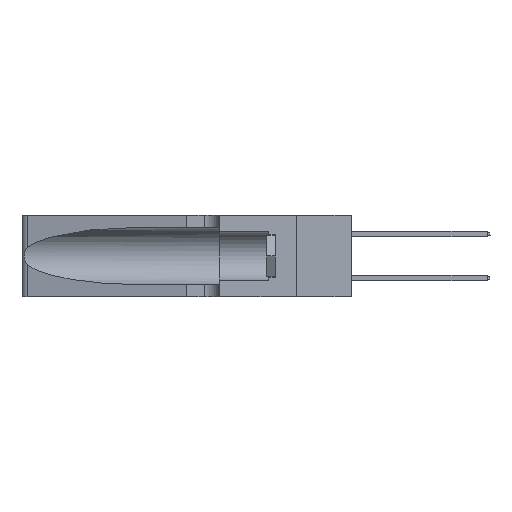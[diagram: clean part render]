
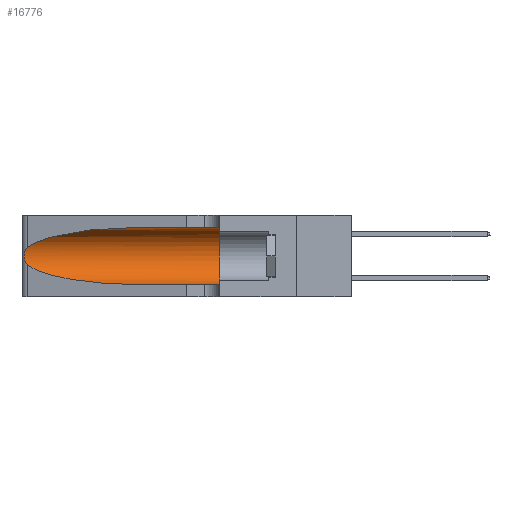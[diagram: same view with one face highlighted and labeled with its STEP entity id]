
A CAD part, left-side view. The second image highlights one B-rep face of the part: STEP entity #16776.
In plain terms, the highlighted cylindrical face has radius 3.308 mm (diameter 6.617 mm), a partial arc.
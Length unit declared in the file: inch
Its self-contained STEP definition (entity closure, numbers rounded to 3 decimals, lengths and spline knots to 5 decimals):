
#282 = EDGE_LOOP ( 'NONE', ( #28429, #18808, #9263, #42537, #4677, #20917 ) ) ;
#328 = CARTESIAN_POINT ( 'NONE',  ( 0.2373, 1.15595, 0.28018 ) ) ;
#1900 = CARTESIAN_POINT ( 'NONE',  ( 0.25487, 1.22718, 0.22369 ) ) ;
#2048 = CARTESIAN_POINT ( 'NONE',  ( 0.25787, 1.23484, 0.2124 ) ) ;
#2056 = VERTEX_POINT ( 'NONE', #17497 ) ;
#2683 = VECTOR ( 'NONE', #10957, 39.37008 ) ;
#3288 = CARTESIAN_POINT ( 'NONE',  ( 0.1305, 1.61858, 0.31525 ) ) ;
#4677 = ORIENTED_EDGE ( 'NONE', *, *, #41355, .F. ) ;
#5514 = CARTESIAN_POINT ( 'NONE',  ( 0.26018, 1.23835, 0.19895 ) ) ;
#6188 = CARTESIAN_POINT ( 'NONE',  ( 0.1305, 0.72297, 0.31525 ) ) ;
#6621 = DIRECTION ( 'NONE',  ( 0., 0., -1. ) ) ;
#8950 = CARTESIAN_POINT ( 'NONE',  ( 0.26075, 1.23896, 0.178 ) ) ;
#9249 = CARTESIAN_POINT ( 'NONE',  ( 0.25487, 1.22718, 0.14631 ) ) ;
#9263 = ORIENTED_EDGE ( 'NONE', *, *, #12343, .T. ) ;
#10132 = CARTESIAN_POINT ( 'NONE',  ( 0.25487, 1.22718, 0.14631 ) ) ;
#10921 = DIRECTION ( 'NONE',  ( 0., 1., 0. ) ) ;
#10957 = DIRECTION ( 'NONE',  ( 0., -1., 0. ) ) ;
#11617 = CARTESIAN_POINT ( 'NONE',  ( 0.1305, 0.35, 0.05475 ) ) ;
#12343 = EDGE_CURVE ( 'NONE', #20862, #30946, #29316, .T. ) ;
#12430 = CARTESIAN_POINT ( 'NONE',  ( 0.25856, 1.23593, 0.16098 ) ) ;
#13592 = CARTESIAN_POINT ( 'NONE',  ( 0.18966, 0.96281, 0.05475 ) ) ;
#14244 = CARTESIAN_POINT ( 'NONE',  ( 0.1305, 0.72297, 0.05475 ) ) ;
#15892 = CARTESIAN_POINT ( 'NONE',  ( 0.25639, 1.23186, 0.15144 ) ) ;
#16776 = ADVANCED_FACE ( 'NONE', ( #23261 ), #31228, .F. ) ;
#17061 = CARTESIAN_POINT ( 'NONE',  ( 0.1305, 0.72297, 0.05475 ) ) ;
#17246 = VECTOR ( 'NONE', #27312, 39.37008 ) ;
#17471 = CARTESIAN_POINT ( 'NONE',  ( 0.18966, 0.96281, 0.31525 ) ) ;
#17497 = CARTESIAN_POINT ( 'NONE',  ( 0.1305, 0.35, 0.31525 ) ) ;
#18808 = ORIENTED_EDGE ( 'NONE', *, *, #31252, .T. ) ;
#19390 = CARTESIAN_POINT ( 'NONE',  ( 0.25487, 1.22718, 0.14631 ) ) ;
#19931 = LINE ( 'NONE', #31491, #2683 ) ;
#20267 = EDGE_CURVE ( 'NONE', #30145, #40987, #33927, .T. ) ;
#20862 = VERTEX_POINT ( 'NONE', #9249 ) ;
#20917 = ORIENTED_EDGE ( 'NONE', *, *, #39255, .F. ) ;
#22650 = CARTESIAN_POINT ( 'NONE',  ( 0.25639, 1.23184, 0.21858 ) ) ;
#23203 = AXIS2_PLACEMENT_3D ( 'NONE', #31457, #10921, #34899 ) ;
#23261 = FACE_OUTER_BOUND ( 'NONE', #282, .T. ) ;
#24356 = CARTESIAN_POINT ( 'NONE',  ( 0.25487, 1.22718, 0.22369 ) ) ;
#26085 = CARTESIAN_POINT ( 'NONE',  ( 0.25854, 1.2359, 0.20912 ) ) ;
#26351 = EDGE_CURVE ( 'NONE', #30946, #40275, #19931, .T. ) ;
#27312 = DIRECTION ( 'NONE',  ( 0., -1., 0. ) ) ;
#28429 = ORIENTED_EDGE ( 'NONE', *, *, #20267, .T. ) ;
#29316 =( BOUNDED_CURVE ( )  B_SPLINE_CURVE ( 3, ( #10132, #30650, #13592, #17061 ),
 .UNSPECIFIED., .F., .F. ) 
 B_SPLINE_CURVE_WITH_KNOTS ( ( 4, 4 ),
 ( 3.44316, 4.71239 ),
 .UNSPECIFIED. ) 
 CURVE ( )  GEOMETRIC_REPRESENTATION_ITEM ( )  RATIONAL_B_SPLINE_CURVE ( ( 1., 0.87, 0.87, 1. ) ) 
 REPRESENTATION_ITEM ( '' )  );
#29510 = CARTESIAN_POINT ( 'NONE',  ( 0.26075, 1.23896, 0.19203 ) ) ;
#30145 = VERTEX_POINT ( 'NONE', #6188 ) ;
#30582 = DIRECTION ( 'NONE',  ( 0., -1., 0. ) ) ;
#30650 = CARTESIAN_POINT ( 'NONE',  ( 0.2373, 1.15595, 0.08982 ) ) ;
#30946 = VERTEX_POINT ( 'NONE', #14244 ) ;
#31228 = CYLINDRICAL_SURFACE ( 'NONE', #35877, 0.13025 ) ;
#31244 = CIRCLE ( 'NONE', #23203, 0.13025 ) ;
#31252 = EDGE_CURVE ( 'NONE', #40987, #20862, #38567, .T. ) ;
#31457 = CARTESIAN_POINT ( 'NONE',  ( 0.1305, 0.35, 0.185 ) ) ;
#31491 = CARTESIAN_POINT ( 'NONE',  ( 0.1305, 1.61858, 0.05475 ) ) ;
#32920 = CARTESIAN_POINT ( 'NONE',  ( 0.26017, 1.23833, 0.17102 ) ) ;
#33927 =( BOUNDED_CURVE ( )  B_SPLINE_CURVE ( 3, ( #41305, #17471, #328, #24356 ),
 .UNSPECIFIED., .F., .T. ) 
 B_SPLINE_CURVE_WITH_KNOTS ( ( 4, 4 ),
 ( 1.5708, 2.84003 ),
 .UNSPECIFIED. ) 
 CURVE ( )  GEOMETRIC_REPRESENTATION_ITEM ( )  RATIONAL_B_SPLINE_CURVE ( ( 1., 0.87, 0.87, 1. ) ) 
 REPRESENTATION_ITEM ( '' )  );
#34021 = CARTESIAN_POINT ( 'NONE',  ( 0.1305, 1.61858, 0.185 ) ) ;
#34899 = DIRECTION ( 'NONE',  ( 0., 0., 1. ) ) ;
#35877 = AXIS2_PLACEMENT_3D ( 'NONE', #34021, #30582, #6621 ) ;
#36330 = CARTESIAN_POINT ( 'NONE',  ( 0.25789, 1.23486, 0.15765 ) ) ;
#38567 = B_SPLINE_CURVE_WITH_KNOTS ( 'NONE', 3,
 ( #1900, #39621, #22650, #2048, #26085, #5514, #29510, #8950, #32920, #12430, #36330, #15892, #39772, #19390 ),
 .UNSPECIFIED., .F., .F.,
 ( 4, 2, 2, 2, 2, 2, 4 ),
 ( 0., 0.00027, 0.00053, 0.00107, 0.0016, 0.00187, 0.00214 ),
 .UNSPECIFIED. ) ;
#39255 = EDGE_CURVE ( 'NONE', #30145, #2056, #43345, .T. ) ;
#39621 = CARTESIAN_POINT ( 'NONE',  ( 0.25555, 1.22994, 0.2215 ) ) ;
#39772 = CARTESIAN_POINT ( 'NONE',  ( 0.25555, 1.22993, 0.14849 ) ) ;
#39836 = CARTESIAN_POINT ( 'NONE',  ( 0.25487, 1.22718, 0.22369 ) ) ;
#40275 = VERTEX_POINT ( 'NONE', #11617 ) ;
#40987 = VERTEX_POINT ( 'NONE', #39836 ) ;
#41305 = CARTESIAN_POINT ( 'NONE',  ( 0.1305, 0.72297, 0.31525 ) ) ;
#41355 = EDGE_CURVE ( 'NONE', #2056, #40275, #31244, .T. ) ;
#42537 = ORIENTED_EDGE ( 'NONE', *, *, #26351, .T. ) ;
#43345 = LINE ( 'NONE', #3288, #17246 ) ;
